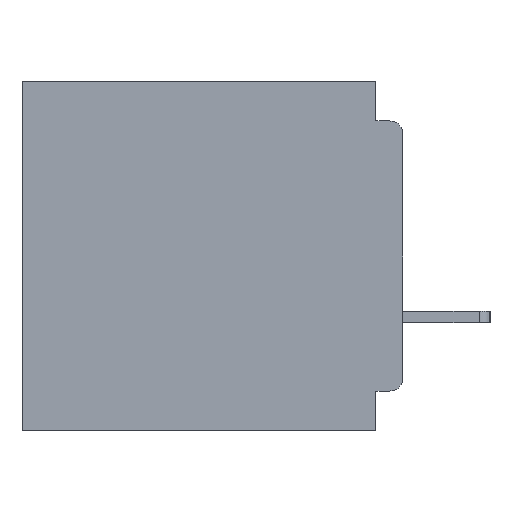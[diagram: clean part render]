
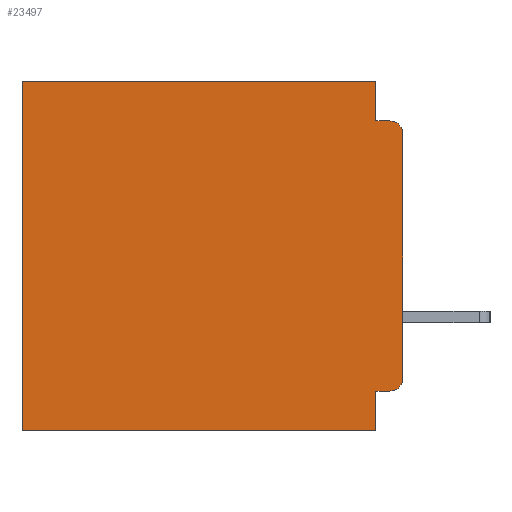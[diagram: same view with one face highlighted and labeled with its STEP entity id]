
A CAD part, left-side view. The second image highlights one B-rep face of the part: STEP entity #23497.
In plain terms, the highlighted planar face has unit normal (-1, 0, 0).
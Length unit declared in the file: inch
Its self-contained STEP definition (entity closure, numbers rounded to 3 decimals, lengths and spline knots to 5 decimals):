
#843 = CARTESIAN_POINT ( 'NONE',  ( 0.3, 0.015, -0.06 ) ) ;
#1413 = CARTESIAN_POINT ( 'NONE',  ( 0.3, 0., -0.06 ) ) ;
#2044 = LINE ( 'NONE', #36299, #10616 ) ;
#2192 = EDGE_CURVE ( 'NONE', #12344, #2347, #8005, .T. ) ;
#2347 = VERTEX_POINT ( 'NONE', #32193 ) ;
#2511 = ORIENTED_EDGE ( 'NONE', *, *, #2192, .F. ) ;
#3093 = DIRECTION ( 'NONE',  ( 0., 1., 0. ) ) ;
#3380 = VERTEX_POINT ( 'NONE', #22981 ) ;
#3439 = AXIS2_PLACEMENT_3D ( 'NONE', #33818, #15148, #36970 ) ;
#3552 = EDGE_CURVE ( 'NONE', #40763, #12344, #2044, .T. ) ;
#4084 = DIRECTION ( 'NONE',  ( 0., 0., -1. ) ) ;
#4486 = CARTESIAN_POINT ( 'NONE',  ( 0.3, 0.031, -0.4 ) ) ;
#5458 = VECTOR ( 'NONE', #30621, 39.37008 ) ;
#5508 = EDGE_CURVE ( 'NONE', #15687, #3380, #6455, .T. ) ;
#6035 = VECTOR ( 'NONE', #6808, 39.37008 ) ;
#6455 = LINE ( 'NONE', #18136, #5458 ) ;
#6740 = FACE_OUTER_BOUND ( 'NONE', #35991, .T. ) ;
#6808 = DIRECTION ( 'NONE',  ( 0., 0., -1. ) ) ;
#7003 = VECTOR ( 'NONE', #26558, 39.37008 ) ;
#7220 = EDGE_CURVE ( 'NONE', #20899, #33179, #14806, .T. ) ;
#7699 = PLANE ( 'NONE',  #38463 ) ;
#8005 = LINE ( 'NONE', #4486, #7003 ) ;
#8944 = VERTEX_POINT ( 'NONE', #21734 ) ;
#8950 = VECTOR ( 'NONE', #27426, 39.37008 ) ;
#9575 = ORIENTED_EDGE ( 'NONE', *, *, #7220, .F. ) ;
#10616 = VECTOR ( 'NONE', #23779, 39.37008 ) ;
#11525 = CARTESIAN_POINT ( 'NONE',  ( 0.3, 0.031, 0. ) ) ;
#11930 = VECTOR ( 'NONE', #28852, 39.37008 ) ;
#12344 = VERTEX_POINT ( 'NONE', #40573 ) ;
#12958 = LINE ( 'NONE', #13303, #11930 ) ;
#13303 = CARTESIAN_POINT ( 'NONE',  ( 0.3, 0., 0. ) ) ;
#13590 = ORIENTED_EDGE ( 'NONE', *, *, #38869, .T. ) ;
#14806 = LINE ( 'NONE', #26988, #31357 ) ;
#15088 = ORIENTED_EDGE ( 'NONE', *, *, #29831, .T. ) ;
#15148 = DIRECTION ( 'NONE',  ( -1., 0., 0. ) ) ;
#15687 = VERTEX_POINT ( 'NONE', #1413 ) ;
#15788 = VERTEX_POINT ( 'NONE', #11525 ) ;
#16415 = CARTESIAN_POINT ( 'NONE',  ( 0.3, 0.437, -0.4 ) ) ;
#17286 = CARTESIAN_POINT ( 'NONE',  ( 0.3, 0., -0.4 ) ) ;
#18136 = CARTESIAN_POINT ( 'NONE',  ( 0.3, 0., -0.4 ) ) ;
#18184 = CARTESIAN_POINT ( 'NONE',  ( 0.3, 0.031, 0. ) ) ;
#18383 = LINE ( 'NONE', #18184, #8950 ) ;
#19586 = CIRCLE ( 'NONE', #3439, 0.015 ) ;
#20433 = DIRECTION ( 'NONE',  ( 0., 0., -1. ) ) ;
#20498 = EDGE_CURVE ( 'NONE', #2347, #8944, #31071, .T. ) ;
#20899 = VERTEX_POINT ( 'NONE', #24413 ) ;
#20953 = ORIENTED_EDGE ( 'NONE', *, *, #21169, .T. ) ;
#21169 = EDGE_CURVE ( 'NONE', #15788, #38621, #12958, .T. ) ;
#21484 = CARTESIAN_POINT ( 'NONE',  ( 0.3, 0.015, -0.045 ) ) ;
#21734 = CARTESIAN_POINT ( 'NONE',  ( 0.3, 0.437, -0.4 ) ) ;
#21867 = LINE ( 'NONE', #16415, #6035 ) ;
#22981 = CARTESIAN_POINT ( 'NONE',  ( 0.3, 0., -0.34 ) ) ;
#23090 = DIRECTION ( 'NONE',  ( -1., 0., 0. ) ) ;
#23497 = ADVANCED_FACE ( 'NONE', ( #6740 ), #7699, .F. ) ;
#23779 = DIRECTION ( 'NONE',  ( 0., 1., 0. ) ) ;
#23812 = VECTOR ( 'NONE', #3093, 39.37008 ) ;
#24019 = DIRECTION ( 'NONE',  ( 0., -1., 0. ) ) ;
#24413 = CARTESIAN_POINT ( 'NONE',  ( 0.3, 0.031, -0.045 ) ) ;
#25260 = CARTESIAN_POINT ( 'NONE',  ( 0.3, 0., -0.4 ) ) ;
#25313 = ORIENTED_EDGE ( 'NONE', *, *, #25807, .T. ) ;
#25807 = EDGE_CURVE ( 'NONE', #15687, #33179, #32649, .T. ) ;
#26558 = DIRECTION ( 'NONE',  ( 0., 0., -1. ) ) ;
#26988 = CARTESIAN_POINT ( 'NONE',  ( 0.3, 0., -0.045 ) ) ;
#27426 = DIRECTION ( 'NONE',  ( 0., 0., -1. ) ) ;
#28852 = DIRECTION ( 'NONE',  ( 0., 1., 0. ) ) ;
#29697 = ORIENTED_EDGE ( 'NONE', *, *, #3552, .F. ) ;
#29831 = EDGE_CURVE ( 'NONE', #40763, #3380, #19586, .T. ) ;
#30621 = DIRECTION ( 'NONE',  ( 0., 0., -1. ) ) ;
#31071 = LINE ( 'NONE', #25260, #23812 ) ;
#31357 = VECTOR ( 'NONE', #24019, 39.37008 ) ;
#31613 = ORIENTED_EDGE ( 'NONE', *, *, #5508, .F. ) ;
#32141 = ORIENTED_EDGE ( 'NONE', *, *, #20498, .F. ) ;
#32193 = CARTESIAN_POINT ( 'NONE',  ( 0.3, 0.031, -0.4 ) ) ;
#32649 = CIRCLE ( 'NONE', #38520, 0.015 ) ;
#33179 = VERTEX_POINT ( 'NONE', #21484 ) ;
#33818 = CARTESIAN_POINT ( 'NONE',  ( 0.3, 0.015, -0.34 ) ) ;
#33888 = CARTESIAN_POINT ( 'NONE',  ( 0.3, 0.015, -0.355 ) ) ;
#34585 = ORIENTED_EDGE ( 'NONE', *, *, #39609, .F. ) ;
#35991 = EDGE_LOOP ( 'NONE', ( #31613, #25313, #9575, #34585, #20953, #13590, #32141, #2511, #29697, #15088 ) ) ;
#36299 = CARTESIAN_POINT ( 'NONE',  ( 0.3, 0., -0.355 ) ) ;
#36970 = DIRECTION ( 'NONE',  ( 0., 0., -1. ) ) ;
#38463 = AXIS2_PLACEMENT_3D ( 'NONE', #17286, #39086, #20433 ) ;
#38520 = AXIS2_PLACEMENT_3D ( 'NONE', #843, #23090, #4084 ) ;
#38621 = VERTEX_POINT ( 'NONE', #40147 ) ;
#38869 = EDGE_CURVE ( 'NONE', #38621, #8944, #21867, .T. ) ;
#39086 = DIRECTION ( 'NONE',  ( 1., 0., 0. ) ) ;
#39609 = EDGE_CURVE ( 'NONE', #15788, #20899, #18383, .T. ) ;
#40147 = CARTESIAN_POINT ( 'NONE',  ( 0.3, 0.437, 0. ) ) ;
#40573 = CARTESIAN_POINT ( 'NONE',  ( 0.3, 0.031, -0.355 ) ) ;
#40763 = VERTEX_POINT ( 'NONE', #33888 ) ;
